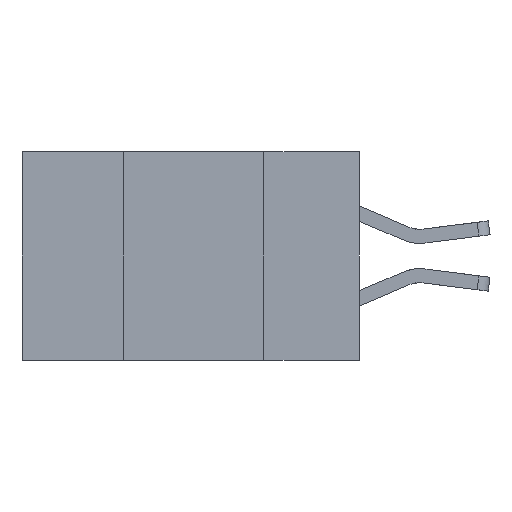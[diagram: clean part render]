
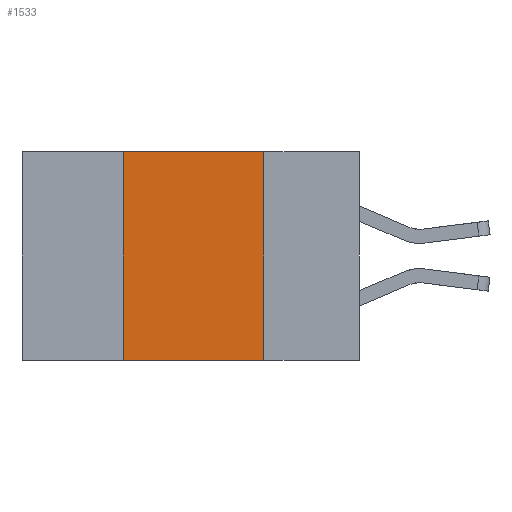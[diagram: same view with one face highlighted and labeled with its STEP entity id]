
A CAD part, left-side view. The second image highlights one B-rep face of the part: STEP entity #1533.
In plain terms, the highlighted planar face has unit normal (-1, 0, 0).
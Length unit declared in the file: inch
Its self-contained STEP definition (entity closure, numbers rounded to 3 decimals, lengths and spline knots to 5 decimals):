
#333 = VECTOR ( 'NONE', #10279, 39.37008 ) ;
#340 = EDGE_CURVE ( 'NONE', #11223, #6482, #11543, .T. ) ;
#962 = PLANE ( 'NONE',  #5232 ) ;
#1423 = CARTESIAN_POINT ( 'NONE',  ( 0., 0.17, -0.37 ) ) ;
#1533 = ADVANCED_FACE ( 'NONE', ( #6586 ), #962, .F. ) ;
#1726 = VECTOR ( 'NONE', #10847, 39.37008 ) ;
#1866 = ORIENTED_EDGE ( 'NONE', *, *, #340, .F. ) ;
#1989 = EDGE_CURVE ( 'NONE', #6482, #9281, #8509, .T. ) ;
#2947 = CARTESIAN_POINT ( 'NONE',  ( 0., 0.6, 0. ) ) ;
#3391 = CARTESIAN_POINT ( 'NONE',  ( 0., 0.17, 0. ) ) ;
#4385 = EDGE_CURVE ( 'NONE', #10853, #11223, #8181, .T. ) ;
#4480 = EDGE_LOOP ( 'NONE', ( #7451, #1866, #8870, #4861 ) ) ;
#4798 = CARTESIAN_POINT ( 'NONE',  ( 0., 0.6, 0. ) ) ;
#4861 = ORIENTED_EDGE ( 'NONE', *, *, #9353, .T. ) ;
#5232 = AXIS2_PLACEMENT_3D ( 'NONE', #4798, #6456, #8458 ) ;
#5363 = CARTESIAN_POINT ( 'NONE',  ( 0., 0.42, 0. ) ) ;
#5436 = LINE ( 'NONE', #11141, #333 ) ;
#6425 = DIRECTION ( 'NONE',  ( 0., 0., 1. ) ) ;
#6456 = DIRECTION ( 'NONE',  ( 1., 0., 0. ) ) ;
#6482 = VERTEX_POINT ( 'NONE', #3391 ) ;
#6586 = FACE_OUTER_BOUND ( 'NONE', #4480, .T. ) ;
#6673 = VECTOR ( 'NONE', #6425, 39.37008 ) ;
#7387 = DIRECTION ( 'NONE',  ( 0., 0., -1. ) ) ;
#7451 = ORIENTED_EDGE ( 'NONE', *, *, #1989, .F. ) ;
#8181 = LINE ( 'NONE', #11261, #6673 ) ;
#8458 = DIRECTION ( 'NONE',  ( 0., 0., -1. ) ) ;
#8509 = LINE ( 'NONE', #12352, #9466 ) ;
#8870 = ORIENTED_EDGE ( 'NONE', *, *, #4385, .F. ) ;
#9281 = VERTEX_POINT ( 'NONE', #1423 ) ;
#9353 = EDGE_CURVE ( 'NONE', #10853, #9281, #5436, .T. ) ;
#9466 = VECTOR ( 'NONE', #7387, 39.37008 ) ;
#10279 = DIRECTION ( 'NONE',  ( 0., -1., 0. ) ) ;
#10642 = CARTESIAN_POINT ( 'NONE',  ( 0., 0.42, -0.37 ) ) ;
#10847 = DIRECTION ( 'NONE',  ( 0., -1., 0. ) ) ;
#10853 = VERTEX_POINT ( 'NONE', #10642 ) ;
#11141 = CARTESIAN_POINT ( 'NONE',  ( 0., 0.6, -0.37 ) ) ;
#11223 = VERTEX_POINT ( 'NONE', #5363 ) ;
#11261 = CARTESIAN_POINT ( 'NONE',  ( 0., 0.42, 0. ) ) ;
#11543 = LINE ( 'NONE', #2947, #1726 ) ;
#12352 = CARTESIAN_POINT ( 'NONE',  ( 0., 0.17, 0. ) ) ;
